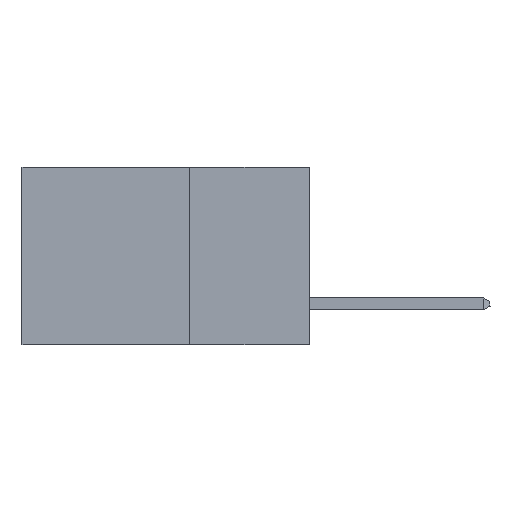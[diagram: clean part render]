
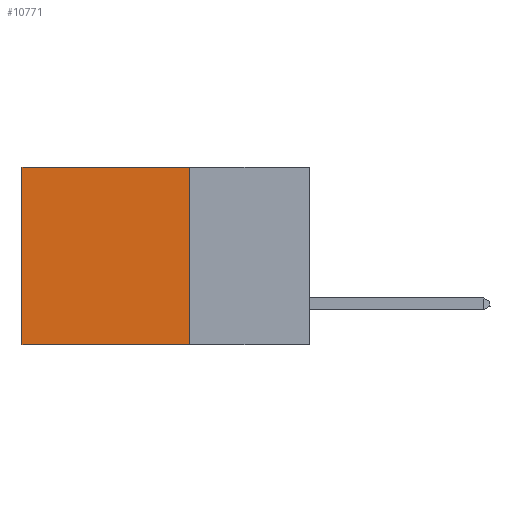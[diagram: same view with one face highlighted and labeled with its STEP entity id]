
A CAD part, left-side view. The second image highlights one B-rep face of the part: STEP entity #10771.
In plain terms, the highlighted planar face has unit normal (-1, 0, 0).
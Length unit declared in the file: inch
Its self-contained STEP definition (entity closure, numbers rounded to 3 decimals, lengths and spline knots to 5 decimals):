
#2386 = EDGE_CURVE ( 'NONE', #4033, #10313, #15284, .T. ) ;
#3230 = CARTESIAN_POINT ( 'NONE',  ( 0.2875, 0.25, 0. ) ) ;
#3602 = CARTESIAN_POINT ( 'NONE',  ( 0.2875, 0.25, -0.37 ) ) ;
#4033 = VERTEX_POINT ( 'NONE', #3230 ) ;
#4479 = EDGE_CURVE ( 'NONE', #10313, #5380, #15415, .T. ) ;
#5154 = LINE ( 'NONE', #10366, #14181 ) ;
#5380 = VERTEX_POINT ( 'NONE', #7074 ) ;
#6213 = DIRECTION ( 'NONE',  ( 1., 0., 0. ) ) ;
#7074 = CARTESIAN_POINT ( 'NONE',  ( 0.2875, 0.6, -0.37 ) ) ;
#7105 = AXIS2_PLACEMENT_3D ( 'NONE', #12778, #6213, #9365 ) ;
#7412 = LINE ( 'NONE', #3602, #10884 ) ;
#8540 = EDGE_LOOP ( 'NONE', ( #15269, #10856, #10322, #15729 ) ) ;
#9113 = DIRECTION ( 'NONE',  ( 0., 0., -1. ) ) ;
#9365 = DIRECTION ( 'NONE',  ( 0., 0., -1. ) ) ;
#9798 = DIRECTION ( 'NONE',  ( 0., 1., 0. ) ) ;
#9844 = CARTESIAN_POINT ( 'NONE',  ( 0.2875, 0.6, 0. ) ) ;
#10313 = VERTEX_POINT ( 'NONE', #14027 ) ;
#10322 = ORIENTED_EDGE ( 'NONE', *, *, #16504, .F. ) ;
#10366 = CARTESIAN_POINT ( 'NONE',  ( 0.2875, 0.25, 0. ) ) ;
#10771 = ADVANCED_FACE ( 'NONE', ( #13170 ), #15504, .F. ) ;
#10856 = ORIENTED_EDGE ( 'NONE', *, *, #12440, .F. ) ;
#10884 = VECTOR ( 'NONE', #16711, 39.37008 ) ;
#12440 = EDGE_CURVE ( 'NONE', #15528, #5380, #7412, .T. ) ;
#12778 = CARTESIAN_POINT ( 'NONE',  ( 0.2875, 0.25, 0. ) ) ;
#13170 = FACE_OUTER_BOUND ( 'NONE', #8540, .T. ) ;
#13469 = CARTESIAN_POINT ( 'NONE',  ( 0.2875, 0.25, 0. ) ) ;
#13989 = DIRECTION ( 'NONE',  ( 0., 0., -1. ) ) ;
#14027 = CARTESIAN_POINT ( 'NONE',  ( 0.2875, 0.6, 0. ) ) ;
#14181 = VECTOR ( 'NONE', #9113, 39.37008 ) ;
#14800 = CARTESIAN_POINT ( 'NONE',  ( 0.2875, 0.25, -0.37 ) ) ;
#14883 = VECTOR ( 'NONE', #9798, 39.37008 ) ;
#15269 = ORIENTED_EDGE ( 'NONE', *, *, #4479, .T. ) ;
#15284 = LINE ( 'NONE', #13469, #14883 ) ;
#15415 = LINE ( 'NONE', #9844, #15627 ) ;
#15504 = PLANE ( 'NONE',  #7105 ) ;
#15528 = VERTEX_POINT ( 'NONE', #14800 ) ;
#15627 = VECTOR ( 'NONE', #13989, 39.37008 ) ;
#15729 = ORIENTED_EDGE ( 'NONE', *, *, #2386, .T. ) ;
#16504 = EDGE_CURVE ( 'NONE', #4033, #15528, #5154, .T. ) ;
#16711 = DIRECTION ( 'NONE',  ( 0., 1., 0. ) ) ;
